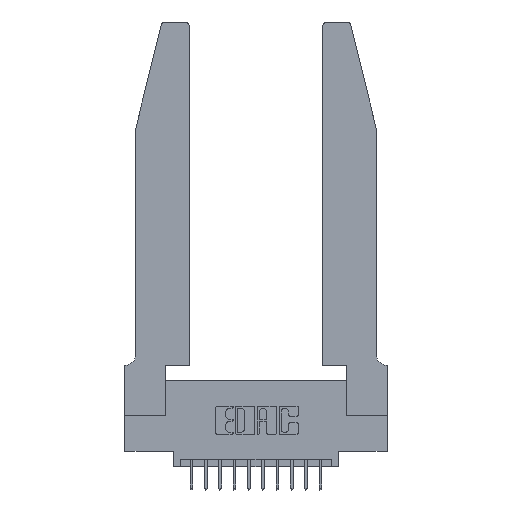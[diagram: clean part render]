
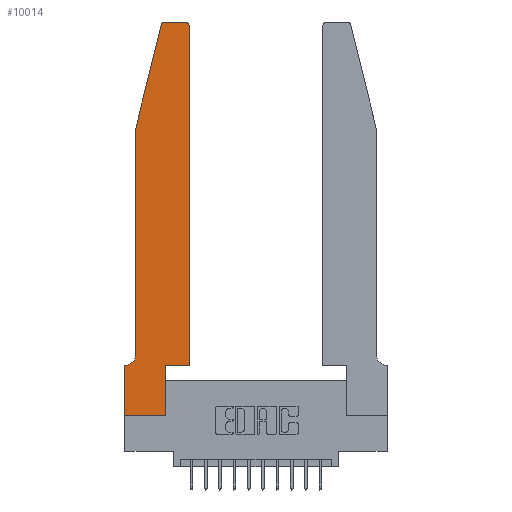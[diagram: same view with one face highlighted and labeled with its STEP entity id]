
A CAD part, top view. The second image highlights one B-rep face of the part: STEP entity #10014.
In plain terms, the highlighted planar face has unit normal (0, 0, 1).
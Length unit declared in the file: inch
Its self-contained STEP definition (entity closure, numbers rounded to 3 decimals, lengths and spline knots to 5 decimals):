
#253 = ORIENTED_EDGE ( 'NONE', *, *, #1968, .T. ) ;
#257 = EDGE_CURVE ( 'NONE', #10544, #5798, #10031, .T. ) ;
#264 = CARTESIAN_POINT ( 'NONE',  ( 0.0055, 0.35, 0.37 ) ) ;
#689 = AXIS2_PLACEMENT_3D ( 'NONE', #3515, #4850, #10110 ) ;
#715 = ORIENTED_EDGE ( 'NONE', *, *, #9905, .T. ) ;
#862 = AXIS2_PLACEMENT_3D ( 'NONE', #2624, #6614, #9291 ) ;
#894 = DIRECTION ( 'NONE',  ( -1., 0., 0. ) ) ;
#1011 = VECTOR ( 'NONE', #15860, 39.37008 ) ;
#1388 = ORIENTED_EDGE ( 'NONE', *, *, #14920, .T. ) ;
#1599 = VECTOR ( 'NONE', #1713, 39.37008 ) ;
#1658 = LINE ( 'NONE', #5292, #9543 ) ;
#1713 = DIRECTION ( 'NONE',  ( -1., 0., 0. ) ) ;
#1950 = VERTEX_POINT ( 'NONE', #4444 ) ;
#1968 = EDGE_CURVE ( 'NONE', #9929, #1950, #11812, .T. ) ;
#2002 = VERTEX_POINT ( 'NONE', #264 ) ;
#2112 = DIRECTION ( 'NONE',  ( 0., 1., 0. ) ) ;
#2216 = ORIENTED_EDGE ( 'NONE', *, *, #15118, .T. ) ;
#2442 = VERTEX_POINT ( 'NONE', #10265 ) ;
#2516 = CIRCLE ( 'NONE', #3781, 0.03 ) ;
#2624 = CARTESIAN_POINT ( 'NONE',  ( 0., 0.35, 0.37 ) ) ;
#2807 = VECTOR ( 'NONE', #13399, 39.37008 ) ;
#3120 = EDGE_CURVE ( 'NONE', #9665, #2442, #12873, .T. ) ;
#3127 = CARTESIAN_POINT ( 'NONE',  ( 0.0755, 2., 0.37 ) ) ;
#3357 = DIRECTION ( 'NONE',  ( 0., 1., 0. ) ) ;
#3515 = CARTESIAN_POINT ( 'NONE',  ( 0.0055, 0.42, 0.37 ) ) ;
#3559 = EDGE_LOOP ( 'NONE', ( #8737, #715, #9547, #15215, #6944, #5552, #253, #5139, #9075, #2216, #16745, #1388 ) ) ;
#3561 = VECTOR ( 'NONE', #8161, 39.37008 ) ;
#3781 = AXIS2_PLACEMENT_3D ( 'NONE', #8492, #12321, #8307 ) ;
#4110 = LINE ( 'NONE', #13435, #1599 ) ;
#4444 = CARTESIAN_POINT ( 'NONE',  ( 0., 0., 0.37 ) ) ;
#4850 = DIRECTION ( 'NONE',  ( 0., 0., -1. ) ) ;
#5139 = ORIENTED_EDGE ( 'NONE', *, *, #15653, .T. ) ;
#5292 = CARTESIAN_POINT ( 'NONE',  ( 0.4505, 0.35, 0.37 ) ) ;
#5300 = PLANE ( 'NONE',  #862 ) ;
#5365 = AXIS2_PLACEMENT_3D ( 'NONE', #14129, #10086, #12673 ) ;
#5552 = ORIENTED_EDGE ( 'NONE', *, *, #17013, .T. ) ;
#5798 = VERTEX_POINT ( 'NONE', #16208 ) ;
#5805 = VECTOR ( 'NONE', #2112, 39.37008 ) ;
#5818 = VECTOR ( 'NONE', #16334, 39.37008 ) ;
#6099 = VECTOR ( 'NONE', #894, 39.37008 ) ;
#6614 = DIRECTION ( 'NONE',  ( 0., 0., 1. ) ) ;
#6616 = LINE ( 'NONE', #11964, #1011 ) ;
#6821 = CARTESIAN_POINT ( 'NONE',  ( 0.25487, 2.72718, 0.37 ) ) ;
#6944 = ORIENTED_EDGE ( 'NONE', *, *, #13666, .T. ) ;
#7465 = CARTESIAN_POINT ( 'NONE',  ( 0.4505, 0.35, 0.37 ) ) ;
#7501 = CARTESIAN_POINT ( 'NONE',  ( 0., 0.35, 0.37 ) ) ;
#7878 = LINE ( 'NONE', #10048, #5805 ) ;
#8161 = DIRECTION ( 'NONE',  ( -0.239, -0.971, 0. ) ) ;
#8203 = CARTESIAN_POINT ( 'NONE',  ( 0.0755, 0.42, 0.37 ) ) ;
#8307 = DIRECTION ( 'NONE',  ( 1., 0., 0. ) ) ;
#8340 = EDGE_CURVE ( 'NONE', #14638, #15665, #14360, .T. ) ;
#8452 = VERTEX_POINT ( 'NONE', #11555 ) ;
#8492 = CARTESIAN_POINT ( 'NONE',  ( 0.284, 2.72, 0.37 ) ) ;
#8737 = ORIENTED_EDGE ( 'NONE', *, *, #257, .T. ) ;
#8786 = CIRCLE ( 'NONE', #689, 0.07 ) ;
#9036 = CARTESIAN_POINT ( 'NONE',  ( 0.2865, 0., 0.37 ) ) ;
#9075 = ORIENTED_EDGE ( 'NONE', *, *, #15925, .T. ) ;
#9291 = DIRECTION ( 'NONE',  ( 1., 0., 0. ) ) ;
#9543 = VECTOR ( 'NONE', #11984, 39.37008 ) ;
#9547 = ORIENTED_EDGE ( 'NONE', *, *, #3120, .T. ) ;
#9600 = CARTESIAN_POINT ( 'NONE',  ( 0., 0., 0.37 ) ) ;
#9665 = VERTEX_POINT ( 'NONE', #6821 ) ;
#9905 = EDGE_CURVE ( 'NONE', #5798, #9665, #2516, .T. ) ;
#9929 = VERTEX_POINT ( 'NONE', #7501 ) ;
#10014 = ADVANCED_FACE ( 'NONE', ( #14100 ), #5300, .T. ) ;
#10031 = LINE ( 'NONE', #16797, #6099 ) ;
#10048 = CARTESIAN_POINT ( 'NONE',  ( 0.2865, 0.35, 0.37 ) ) ;
#10086 = DIRECTION ( 'NONE',  ( 0., 0., 1. ) ) ;
#10110 = DIRECTION ( 'NONE',  ( -1., 0., 0. ) ) ;
#10265 = CARTESIAN_POINT ( 'NONE',  ( 0.0755, 2., 0.37 ) ) ;
#10544 = VERTEX_POINT ( 'NONE', #16932 ) ;
#11269 = VERTEX_POINT ( 'NONE', #8203 ) ;
#11555 = CARTESIAN_POINT ( 'NONE',  ( 0.2865, 0.35, 0.37 ) ) ;
#11700 = LINE ( 'NONE', #13521, #2807 ) ;
#11812 = LINE ( 'NONE', #9600, #5818 ) ;
#11964 = CARTESIAN_POINT ( 'NONE',  ( 0., 0., 0.37 ) ) ;
#11984 = DIRECTION ( 'NONE',  ( 1., 0., 0. ) ) ;
#12018 = CARTESIAN_POINT ( 'NONE',  ( 0.4505, 2.72, 0.37 ) ) ;
#12321 = DIRECTION ( 'NONE',  ( 0., 0., 1. ) ) ;
#12631 = CIRCLE ( 'NONE', #5365, 0.03 ) ;
#12655 = EDGE_CURVE ( 'NONE', #2442, #11269, #11700, .T. ) ;
#12673 = DIRECTION ( 'NONE',  ( 1., 0., 0. ) ) ;
#12873 = LINE ( 'NONE', #3127, #3561 ) ;
#13355 = CARTESIAN_POINT ( 'NONE',  ( 0.4505, 0.35, 0.37 ) ) ;
#13399 = DIRECTION ( 'NONE',  ( 0., -1., 0. ) ) ;
#13435 = CARTESIAN_POINT ( 'NONE',  ( 0.0755, 0.35, 0.37 ) ) ;
#13521 = CARTESIAN_POINT ( 'NONE',  ( 0.0755, 2., 0.37 ) ) ;
#13666 = EDGE_CURVE ( 'NONE', #11269, #2002, #8786, .T. ) ;
#14100 = FACE_OUTER_BOUND ( 'NONE', #3559, .T. ) ;
#14129 = CARTESIAN_POINT ( 'NONE',  ( 0.4205, 2.72, 0.37 ) ) ;
#14360 = LINE ( 'NONE', #7465, #14766 ) ;
#14638 = VERTEX_POINT ( 'NONE', #13355 ) ;
#14766 = VECTOR ( 'NONE', #3357, 39.37008 ) ;
#14920 = EDGE_CURVE ( 'NONE', #15665, #10544, #12631, .T. ) ;
#15118 = EDGE_CURVE ( 'NONE', #8452, #14638, #1658, .T. ) ;
#15215 = ORIENTED_EDGE ( 'NONE', *, *, #12655, .T. ) ;
#15653 = EDGE_CURVE ( 'NONE', #1950, #16786, #6616, .T. ) ;
#15665 = VERTEX_POINT ( 'NONE', #12018 ) ;
#15860 = DIRECTION ( 'NONE',  ( 1., 0., 0. ) ) ;
#15925 = EDGE_CURVE ( 'NONE', #16786, #8452, #7878, .T. ) ;
#16208 = CARTESIAN_POINT ( 'NONE',  ( 0.284, 2.75, 0.37 ) ) ;
#16334 = DIRECTION ( 'NONE',  ( 0., -1., 0. ) ) ;
#16745 = ORIENTED_EDGE ( 'NONE', *, *, #8340, .T. ) ;
#16786 = VERTEX_POINT ( 'NONE', #9036 ) ;
#16797 = CARTESIAN_POINT ( 'NONE',  ( 0.2605, 2.75, 0.37 ) ) ;
#16932 = CARTESIAN_POINT ( 'NONE',  ( 0.4205, 2.75, 0.37 ) ) ;
#17013 = EDGE_CURVE ( 'NONE', #2002, #9929, #4110, .T. ) ;
